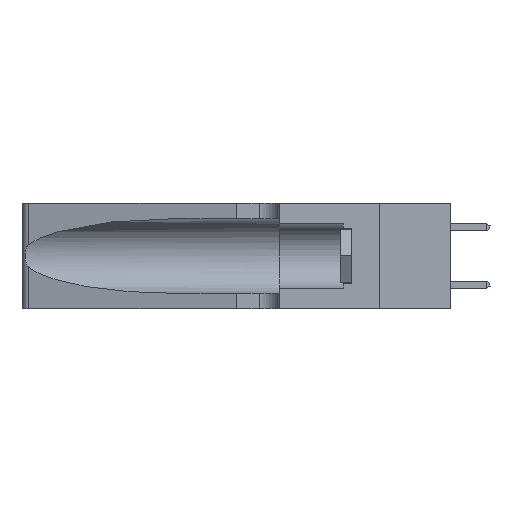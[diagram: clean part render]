
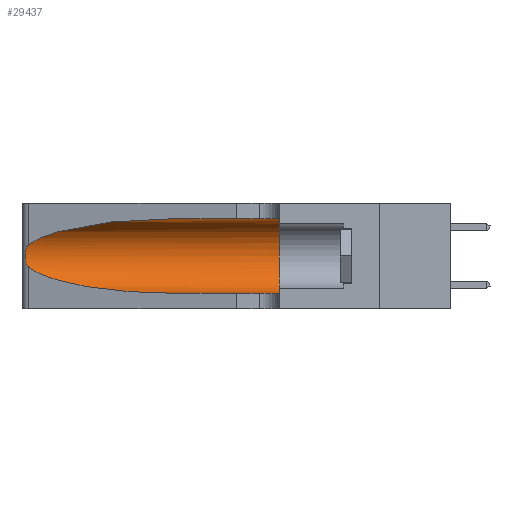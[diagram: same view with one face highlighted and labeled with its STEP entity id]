
A CAD part, left-side view. The second image highlights one B-rep face of the part: STEP entity #29437.
In plain terms, the highlighted cylindrical face has radius 3.308 mm (diameter 6.617 mm), a partial arc.
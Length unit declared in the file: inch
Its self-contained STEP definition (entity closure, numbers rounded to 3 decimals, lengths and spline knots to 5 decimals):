
#481 = CARTESIAN_POINT ( 'NONE',  ( 0.25555, 1.22994, 0.2215 ) ) ;
#692 = EDGE_CURVE ( 'NONE', #19597, #21365, #36179, .T. ) ;
#1339 = CARTESIAN_POINT ( 'NONE',  ( 0.1305, 1.61858, 0.185 ) ) ;
#2764 = CARTESIAN_POINT ( 'NONE',  ( 0.25487, 1.22718, 0.22369 ) ) ;
#2929 = ORIENTED_EDGE ( 'NONE', *, *, #7836, .T. ) ;
#2983 = CARTESIAN_POINT ( 'NONE',  ( 0.18966, 0.96281, 0.31525 ) ) ;
#3150 = CARTESIAN_POINT ( 'NONE',  ( 0.26018, 1.23835, 0.19895 ) ) ;
#3279 = CARTESIAN_POINT ( 'NONE',  ( 0.26075, 1.23896, 0.19203 ) ) ;
#3642 = EDGE_CURVE ( 'NONE', #7806, #19597, #6149, .T. ) ;
#4799 = CARTESIAN_POINT ( 'NONE',  ( 0.1305, 0.72297, 0.31525 ) ) ;
#5436 = LINE ( 'NONE', #25565, #35155 ) ;
#6149 = LINE ( 'NONE', #33956, #29782 ) ;
#6277 = CARTESIAN_POINT ( 'NONE',  ( 0.25789, 1.23486, 0.15765 ) ) ;
#6646 = CARTESIAN_POINT ( 'NONE',  ( 0.25487, 1.22718, 0.14631 ) ) ;
#7245 = EDGE_CURVE ( 'NONE', #16507, #21365, #5436, .T. ) ;
#7806 = VERTEX_POINT ( 'NONE', #4799 ) ;
#7832 = CARTESIAN_POINT ( 'NONE',  ( 0.25487, 1.22718, 0.14631 ) ) ;
#7836 = EDGE_CURVE ( 'NONE', #31206, #16507, #7944, .T. ) ;
#7944 =( BOUNDED_CURVE ( )  B_SPLINE_CURVE ( 3, ( #7832, #35138, #23264, #29346 ),
 .UNSPECIFIED., .F., .F. ) 
 B_SPLINE_CURVE_WITH_KNOTS ( ( 4, 4 ),
 ( 3.44316, 4.71239 ),
 .UNSPECIFIED. ) 
 CURVE ( )  GEOMETRIC_REPRESENTATION_ITEM ( )  RATIONAL_B_SPLINE_CURVE ( ( 1., 0.87, 0.87, 1. ) ) 
 REPRESENTATION_ITEM ( '' )  );
#8444 = B_SPLINE_CURVE_WITH_KNOTS ( 'NONE', 3,
 ( #30814, #481, #21314, #12603, #30553, #3150, #3279, #33706, #36749, #24372, #6277, #27385, #21186, #6646 ),
 .UNSPECIFIED., .F., .F.,
 ( 4, 2, 2, 2, 2, 2, 4 ),
 ( 0., 0.00027, 0.00053, 0.00107, 0.0016, 0.00187, 0.00214 ),
 .UNSPECIFIED. ) ;
#9268 = VERTEX_POINT ( 'NONE', #2764 ) ;
#10236 = ORIENTED_EDGE ( 'NONE', *, *, #15699, .T. ) ;
#10407 = DIRECTION ( 'NONE',  ( 0., -1., 0. ) ) ;
#11675 = CARTESIAN_POINT ( 'NONE',  ( 0.1305, 0.72297, 0.31525 ) ) ;
#12029 = DIRECTION ( 'NONE',  ( 0., 1., 0. ) ) ;
#12603 = CARTESIAN_POINT ( 'NONE',  ( 0.25787, 1.23484, 0.2124 ) ) ;
#12779 = CARTESIAN_POINT ( 'NONE',  ( 0.25487, 1.22718, 0.14631 ) ) ;
#13316 = CYLINDRICAL_SURFACE ( 'NONE', #30249, 0.13025 ) ;
#13814 = ORIENTED_EDGE ( 'NONE', *, *, #34057, .T. ) ;
#14239 = CARTESIAN_POINT ( 'NONE',  ( 0.1305, 0.72297, 0.05475 ) ) ;
#15699 = EDGE_CURVE ( 'NONE', #7806, #9268, #35310, .T. ) ;
#16507 = VERTEX_POINT ( 'NONE', #14239 ) ;
#16601 = FACE_OUTER_BOUND ( 'NONE', #30353, .T. ) ;
#18445 = CARTESIAN_POINT ( 'NONE',  ( 0.1305, 0.35, 0.185 ) ) ;
#19597 = VERTEX_POINT ( 'NONE', #30811 ) ;
#19664 = ORIENTED_EDGE ( 'NONE', *, *, #7245, .T. ) ;
#21186 = CARTESIAN_POINT ( 'NONE',  ( 0.25555, 1.22993, 0.14849 ) ) ;
#21314 = CARTESIAN_POINT ( 'NONE',  ( 0.25639, 1.23184, 0.21858 ) ) ;
#21365 = VERTEX_POINT ( 'NONE', #25610 ) ;
#23264 = CARTESIAN_POINT ( 'NONE',  ( 0.18966, 0.96281, 0.05475 ) ) ;
#24372 = CARTESIAN_POINT ( 'NONE',  ( 0.25856, 1.23593, 0.16098 ) ) ;
#25565 = CARTESIAN_POINT ( 'NONE',  ( 0.1305, 1.61858, 0.05475 ) ) ;
#25610 = CARTESIAN_POINT ( 'NONE',  ( 0.1305, 0.35, 0.05475 ) ) ;
#25940 = DIRECTION ( 'NONE',  ( 0., 0., -1. ) ) ;
#26220 = DIRECTION ( 'NONE',  ( 0., -1., 0. ) ) ;
#26562 = DIRECTION ( 'NONE',  ( 0., 0., 1. ) ) ;
#27385 = CARTESIAN_POINT ( 'NONE',  ( 0.25639, 1.23186, 0.15144 ) ) ;
#29346 = CARTESIAN_POINT ( 'NONE',  ( 0.1305, 0.72297, 0.05475 ) ) ;
#29437 = ADVANCED_FACE ( 'NONE', ( #16601 ), #13316, .F. ) ;
#29782 = VECTOR ( 'NONE', #26220, 39.37008 ) ;
#29965 = ORIENTED_EDGE ( 'NONE', *, *, #3642, .F. ) ;
#30249 = AXIS2_PLACEMENT_3D ( 'NONE', #1339, #10407, #25940 ) ;
#30353 = EDGE_LOOP ( 'NONE', ( #10236, #13814, #2929, #19664, #38537, #29965 ) ) ;
#30553 = CARTESIAN_POINT ( 'NONE',  ( 0.25854, 1.2359, 0.20912 ) ) ;
#30811 = CARTESIAN_POINT ( 'NONE',  ( 0.1305, 0.35, 0.31525 ) ) ;
#30814 = CARTESIAN_POINT ( 'NONE',  ( 0.25487, 1.22718, 0.22369 ) ) ;
#31206 = VERTEX_POINT ( 'NONE', #12779 ) ;
#32029 = DIRECTION ( 'NONE',  ( 0., -1., 0. ) ) ;
#32667 = AXIS2_PLACEMENT_3D ( 'NONE', #18445, #12029, #26562 ) ;
#32783 = CARTESIAN_POINT ( 'NONE',  ( 0.2373, 1.15595, 0.28018 ) ) ;
#33706 = CARTESIAN_POINT ( 'NONE',  ( 0.26075, 1.23896, 0.178 ) ) ;
#33956 = CARTESIAN_POINT ( 'NONE',  ( 0.1305, 1.61858, 0.31525 ) ) ;
#34057 = EDGE_CURVE ( 'NONE', #9268, #31206, #8444, .T. ) ;
#35138 = CARTESIAN_POINT ( 'NONE',  ( 0.2373, 1.15595, 0.08982 ) ) ;
#35155 = VECTOR ( 'NONE', #32029, 39.37008 ) ;
#35310 =( BOUNDED_CURVE ( )  B_SPLINE_CURVE ( 3, ( #11675, #2983, #32783, #38836 ),
 .UNSPECIFIED., .F., .T. ) 
 B_SPLINE_CURVE_WITH_KNOTS ( ( 4, 4 ),
 ( 1.5708, 2.84003 ),
 .UNSPECIFIED. ) 
 CURVE ( )  GEOMETRIC_REPRESENTATION_ITEM ( )  RATIONAL_B_SPLINE_CURVE ( ( 1., 0.87, 0.87, 1. ) ) 
 REPRESENTATION_ITEM ( '' )  );
#36179 = CIRCLE ( 'NONE', #32667, 0.13025 ) ;
#36749 = CARTESIAN_POINT ( 'NONE',  ( 0.26017, 1.23833, 0.17102 ) ) ;
#38537 = ORIENTED_EDGE ( 'NONE', *, *, #692, .F. ) ;
#38836 = CARTESIAN_POINT ( 'NONE',  ( 0.25487, 1.22718, 0.22369 ) ) ;
